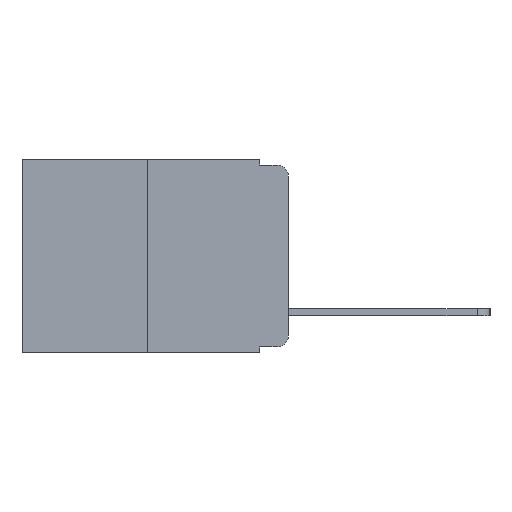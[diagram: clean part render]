
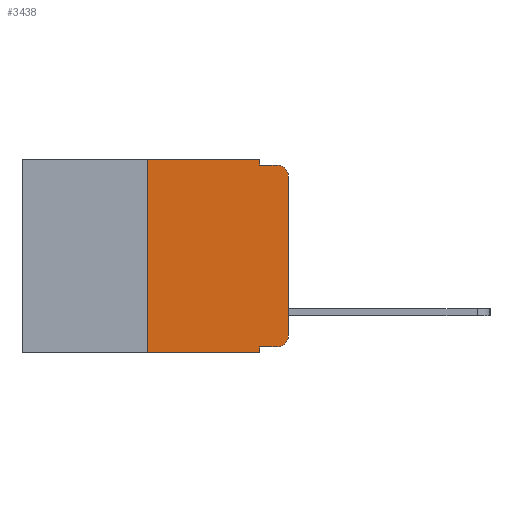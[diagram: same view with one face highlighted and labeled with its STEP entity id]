
A CAD part, left-side view. The second image highlights one B-rep face of the part: STEP entity #3438.
In plain terms, the highlighted planar face has unit normal (-1, 0, 0).
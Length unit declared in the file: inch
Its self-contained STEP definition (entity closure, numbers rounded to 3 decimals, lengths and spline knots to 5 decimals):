
#163 = DIRECTION ( 'NONE',  ( 0., -1., 0. ) ) ;
#192 = AXIS2_PLACEMENT_3D ( 'NONE', #1506, #10190, #2218 ) ;
#412 = AXIS2_PLACEMENT_3D ( 'NONE', #6530, #14989, #7742 ) ;
#456 = VECTOR ( 'NONE', #8089, 39.37008 ) ;
#879 = EDGE_CURVE ( 'NONE', #1669, #2022, #5822, .T. ) ;
#1021 = EDGE_CURVE ( 'NONE', #12140, #5004, #13961, .T. ) ;
#1160 = ORIENTED_EDGE ( 'NONE', *, *, #10595, .T. ) ;
#1329 = EDGE_LOOP ( 'NONE', ( #5514, #9638, #3374, #12673, #13703, #10788, #10055, #15302, #7399, #1160 ) ) ;
#1506 = CARTESIAN_POINT ( 'NONE',  ( 0., 0.473, 0. ) ) ;
#1625 = CARTESIAN_POINT ( 'NONE',  ( 0., 0.473, 0. ) ) ;
#1669 = VERTEX_POINT ( 'NONE', #7624 ) ;
#1948 = VECTOR ( 'NONE', #11475, 39.37008 ) ;
#2022 = VERTEX_POINT ( 'NONE', #11270 ) ;
#2218 = DIRECTION ( 'NONE',  ( 0., 0., -1. ) ) ;
#2552 = CARTESIAN_POINT ( 'NONE',  ( 0., 0.051, -0.343 ) ) ;
#3374 = ORIENTED_EDGE ( 'NONE', *, *, #879, .F. ) ;
#3438 = ADVANCED_FACE ( 'NONE', ( #12402 ), #15675, .F. ) ;
#3482 = CIRCLE ( 'NONE', #412, 0.02 ) ;
#3813 = AXIS2_PLACEMENT_3D ( 'NONE', #4705, #13273, #6014 ) ;
#3955 = EDGE_CURVE ( 'NONE', #5004, #1669, #12003, .T. ) ;
#4021 = VERTEX_POINT ( 'NONE', #7020 ) ;
#4030 = VECTOR ( 'NONE', #6541, 39.37008 ) ;
#4179 = VECTOR ( 'NONE', #9387, 39.37008 ) ;
#4378 = EDGE_CURVE ( 'NONE', #8972, #11217, #12759, .T. ) ;
#4705 = CARTESIAN_POINT ( 'NONE',  ( 0., 0.02, -0.313 ) ) ;
#5004 = VERTEX_POINT ( 'NONE', #12664 ) ;
#5157 = LINE ( 'NONE', #12499, #11252 ) ;
#5286 = CARTESIAN_POINT ( 'NONE',  ( 0., 0.25, 0. ) ) ;
#5355 = DIRECTION ( 'NONE',  ( 0., -1., 0. ) ) ;
#5514 = ORIENTED_EDGE ( 'NONE', *, *, #13121, .T. ) ;
#5545 = VECTOR ( 'NONE', #8436, 39.37008 ) ;
#5822 = LINE ( 'NONE', #8621, #6210 ) ;
#6014 = DIRECTION ( 'NONE',  ( 0., 0., -1. ) ) ;
#6082 = CARTESIAN_POINT ( 'NONE',  ( 0., 0.473, -0.343 ) ) ;
#6210 = VECTOR ( 'NONE', #163, 39.37008 ) ;
#6528 = DIRECTION ( 'NONE',  ( 0., 0., 1. ) ) ;
#6530 = CARTESIAN_POINT ( 'NONE',  ( 0., 0.02, -0.03 ) ) ;
#6541 = DIRECTION ( 'NONE',  ( 0., 0., 1. ) ) ;
#6811 = CARTESIAN_POINT ( 'NONE',  ( 0., 0.051, -0.333 ) ) ;
#6876 = CARTESIAN_POINT ( 'NONE',  ( 0., 0.051, -0.333 ) ) ;
#7020 = CARTESIAN_POINT ( 'NONE',  ( 0., 0.02, -0.333 ) ) ;
#7338 = EDGE_CURVE ( 'NONE', #8972, #12140, #13827, .T. ) ;
#7399 = ORIENTED_EDGE ( 'NONE', *, *, #9773, .T. ) ;
#7624 = CARTESIAN_POINT ( 'NONE',  ( 0., 0.051, -0.01 ) ) ;
#7694 = CARTESIAN_POINT ( 'NONE',  ( 0., 0.25, -0.343 ) ) ;
#7742 = DIRECTION ( 'NONE',  ( 0., 0., -1. ) ) ;
#7747 = CARTESIAN_POINT ( 'NONE',  ( 0., 0., -0.03 ) ) ;
#7947 = LINE ( 'NONE', #6876, #456 ) ;
#8089 = DIRECTION ( 'NONE',  ( 0., -1., 0. ) ) ;
#8146 = EDGE_CURVE ( 'NONE', #11992, #11217, #11232, .T. ) ;
#8436 = DIRECTION ( 'NONE',  ( 0., 0., -1. ) ) ;
#8621 = CARTESIAN_POINT ( 'NONE',  ( 0., 0.051, -0.01 ) ) ;
#8972 = VERTEX_POINT ( 'NONE', #7694 ) ;
#9003 = VERTEX_POINT ( 'NONE', #7747 ) ;
#9387 = DIRECTION ( 'NONE',  ( 0., -1., 0. ) ) ;
#9424 = CARTESIAN_POINT ( 'NONE',  ( 0., 0., -0.313 ) ) ;
#9638 = ORIENTED_EDGE ( 'NONE', *, *, #16311, .T. ) ;
#9773 = EDGE_CURVE ( 'NONE', #11992, #4021, #7947, .T. ) ;
#10055 = ORIENTED_EDGE ( 'NONE', *, *, #4378, .T. ) ;
#10190 = DIRECTION ( 'NONE',  ( 1., 0., 0. ) ) ;
#10595 = EDGE_CURVE ( 'NONE', #4021, #13564, #13982, .T. ) ;
#10788 = ORIENTED_EDGE ( 'NONE', *, *, #7338, .F. ) ;
#11217 = VERTEX_POINT ( 'NONE', #2552 ) ;
#11232 = LINE ( 'NONE', #14497, #5545 ) ;
#11252 = VECTOR ( 'NONE', #6528, 39.37008 ) ;
#11270 = CARTESIAN_POINT ( 'NONE',  ( 0., 0.02, -0.01 ) ) ;
#11475 = DIRECTION ( 'NONE',  ( 0., 0., -1. ) ) ;
#11945 = CARTESIAN_POINT ( 'NONE',  ( 0., 0.25, 0. ) ) ;
#11992 = VERTEX_POINT ( 'NONE', #6811 ) ;
#12003 = LINE ( 'NONE', #13959, #1948 ) ;
#12140 = VERTEX_POINT ( 'NONE', #11945 ) ;
#12402 = FACE_OUTER_BOUND ( 'NONE', #1329, .T. ) ;
#12499 = CARTESIAN_POINT ( 'NONE',  ( 0., 0., 0. ) ) ;
#12664 = CARTESIAN_POINT ( 'NONE',  ( 0., 0.051, 0. ) ) ;
#12673 = ORIENTED_EDGE ( 'NONE', *, *, #3955, .F. ) ;
#12759 = LINE ( 'NONE', #6082, #15556 ) ;
#13121 = EDGE_CURVE ( 'NONE', #13564, #9003, #5157, .T. ) ;
#13273 = DIRECTION ( 'NONE',  ( -1., 0., 0. ) ) ;
#13564 = VERTEX_POINT ( 'NONE', #9424 ) ;
#13703 = ORIENTED_EDGE ( 'NONE', *, *, #1021, .F. ) ;
#13827 = LINE ( 'NONE', #5286, #4030 ) ;
#13959 = CARTESIAN_POINT ( 'NONE',  ( 0., 0.051, 0. ) ) ;
#13961 = LINE ( 'NONE', #1625, #4179 ) ;
#13982 = CIRCLE ( 'NONE', #3813, 0.02 ) ;
#14497 = CARTESIAN_POINT ( 'NONE',  ( 0., 0.051, 0. ) ) ;
#14989 = DIRECTION ( 'NONE',  ( -1., 0., 0. ) ) ;
#15302 = ORIENTED_EDGE ( 'NONE', *, *, #8146, .F. ) ;
#15556 = VECTOR ( 'NONE', #5355, 39.37008 ) ;
#15675 = PLANE ( 'NONE',  #192 ) ;
#16311 = EDGE_CURVE ( 'NONE', #9003, #2022, #3482, .T. ) ;
